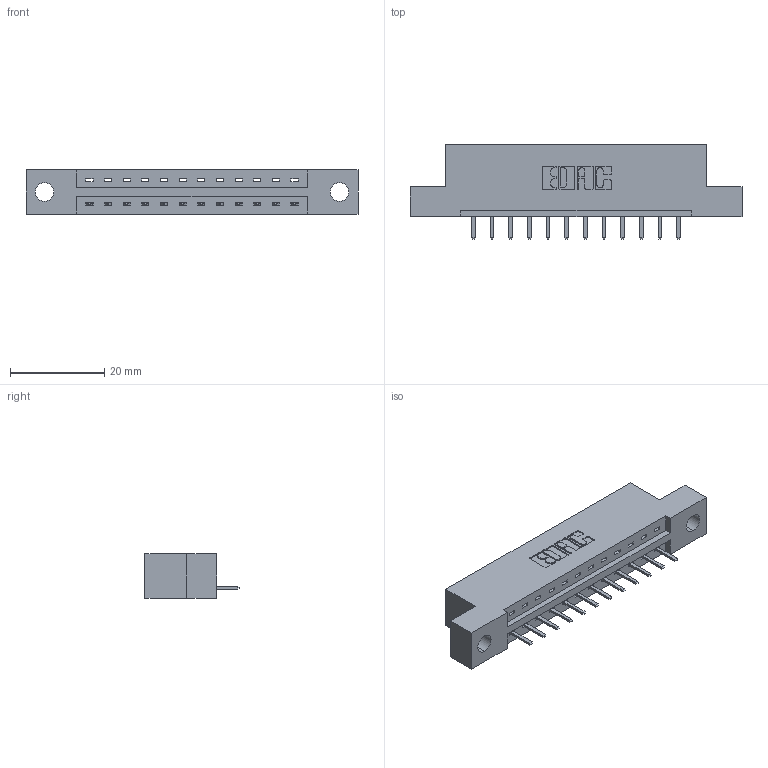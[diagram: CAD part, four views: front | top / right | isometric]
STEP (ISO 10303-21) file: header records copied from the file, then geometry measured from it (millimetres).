
FILE_DESCRIPTION (( 'STEP AP203' ), '1' );
FILE_NAME ('387-012-520-104.STEP', '2019-10-02T12:47:27', ( '' ), ( '' ), 'SwSTEP 2.0', 'SolidWorks 2016', '' );
FILE_SCHEMA (( 'CONFIG_CONTROL_DESIGN' ));
Length unit declared in the file: inch
Products named in the file (3): 345-292-001_345-293-120; 387-012-520-104; 337 Part_Flush Mounting Lugs - 0.156 Dia-TH
Assembly tree (13 placements, depth 2):
  387-012-520-104
    337 Part_Flush Mounting Lugs - 0.156 Dia-TH
    345-292-001_345-293-120  x12
Bounding box: 70.56 x 20.02 x 9.4 mm (x, y, z)
Volume: 6835.9 mm3; surface area: 6568.4 mm2
Topology: 13 solids, 13 shells, 906 faces, 2663 edges, 1742 vertices
Faces by surface type: plane 646, cylinder 260
Entity records: 12917 total; most frequent: CARTESIAN_POINT 2266, ORIENTED_EDGE 2202, DIRECTION 1957, EDGE_CURVE 1101, VECTOR 969, LINE 969, VERTEX_POINT 730, AXIS2_PLACEMENT_3D 494
